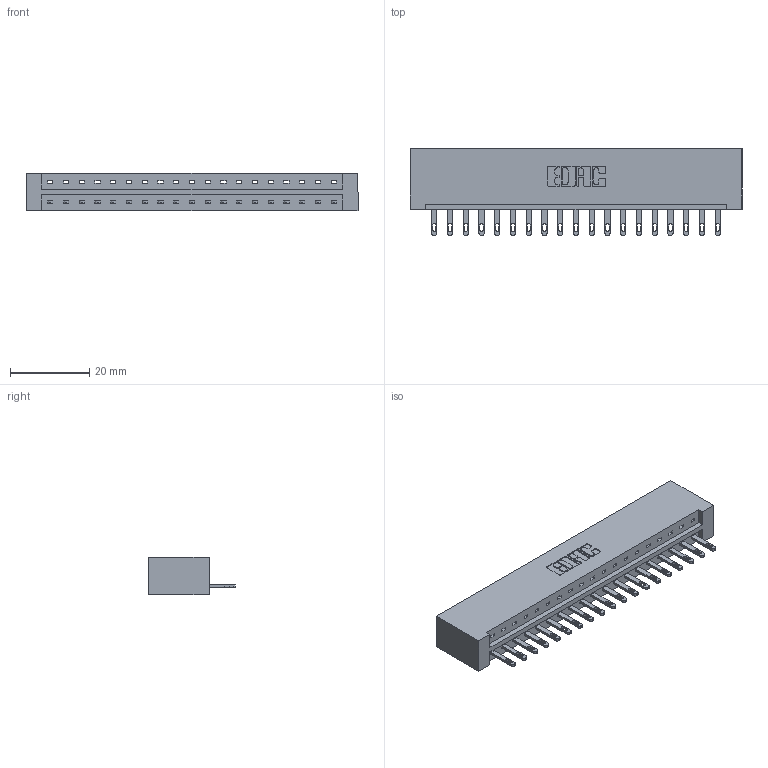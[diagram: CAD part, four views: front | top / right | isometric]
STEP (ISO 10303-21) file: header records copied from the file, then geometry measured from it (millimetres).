
FILE_DESCRIPTION (( 'STEP AP203' ), '1' );
FILE_NAME ('333-019-500-101.STEP', '2018-08-01T22:56:55', ( '' ), ( '' ), 'SwSTEP 2.0', 'SolidWorks 2016', '' );
FILE_SCHEMA (( 'CONFIG_CONTROL_DESIGN' ));
Length unit declared in the file: inch
Products named in the file (3): 333 Part_Lugless; 345-292-001_345-293-100; 333-019-500-101
Assembly tree (20 placements, depth 2):
  333-019-500-101
    333 Part_Lugless
    345-292-001_345-293-100  x19
Bounding box: 83.54 x 21.85 x 9.4 mm (x, y, z)
Volume: 8833.3 mm3; surface area: 9409.5 mm2
Topology: 20 solids, 20 shells, 1132 faces, 3479 edges, 2318 vertices
Faces by surface type: plane 750, cylinder 382
Entity records: 14243 total; most frequent: CARTESIAN_POINT 2467, ORIENTED_EDGE 2422, DIRECTION 2121, EDGE_CURVE 1211, LINE 1087, VECTOR 1087, VERTEX_POINT 806, AXIS2_PLACEMENT_3D 517
